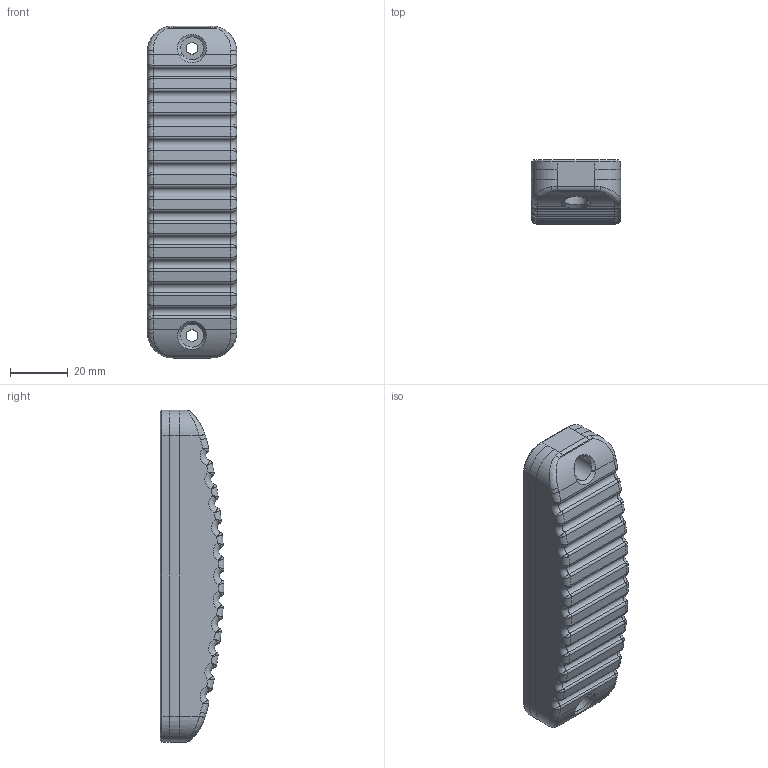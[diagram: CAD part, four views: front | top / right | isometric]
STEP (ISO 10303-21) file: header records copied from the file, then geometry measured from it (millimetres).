
FILE_DESCRIPTION(/* description */ (''),/* implementation_level */ '2;1');
FILE_NAME(/* name */ 'Convex Buttpad.step',/* time_stamp */ '2021-07-28T09:04:06-04:00',/* author */ (''),/* organization */ (''),/* preprocessor_version */ 'ST-DEVELOPER v18.1',/* originating_system */ 'Autodesk Translation Framework v10.9.0.1377',/* authorisation */ '');
FILE_SCHEMA (('AUTOMOTIVE_DESIGN { 1 0 10303 214 3 1 1 }'));
Length unit declared in the file: millimetre
Products named in the file (1): Convex Buttpad
Bounding box: 31 x 22.15 x 115 mm (x, y, z)
Volume: 64115.1 mm3; surface area: 12468.3 mm2
Topology: 1 solids, 1 shells, 202 faces, 474 edges, 230 vertices
Faces by surface type: bspline 68, cylinder 61, torus 58, plane 13, cone 2
Full cylindrical faces by diameter (mm): 4 x2, 8 x2
Entity records: 9723 total; most frequent: CARTESIAN_POINT 5708, ORIENTED_EDGE 860, DIRECTION 770, EDGE_CURVE 430, AXIS2_PLACEMENT_3D 335, VERTEX_POINT 230, EDGE_LOOP 206, FACE_OUTER_BOUND 202
